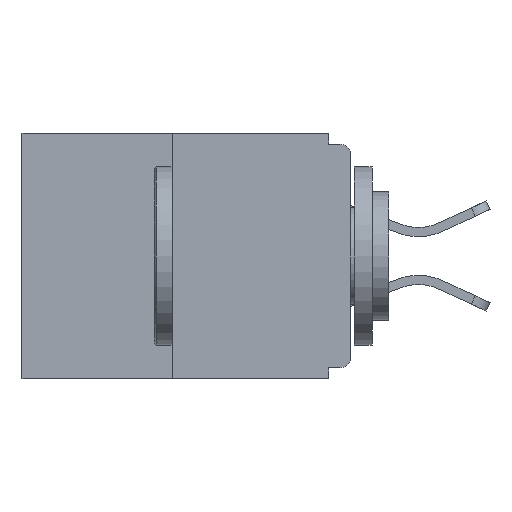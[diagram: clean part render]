
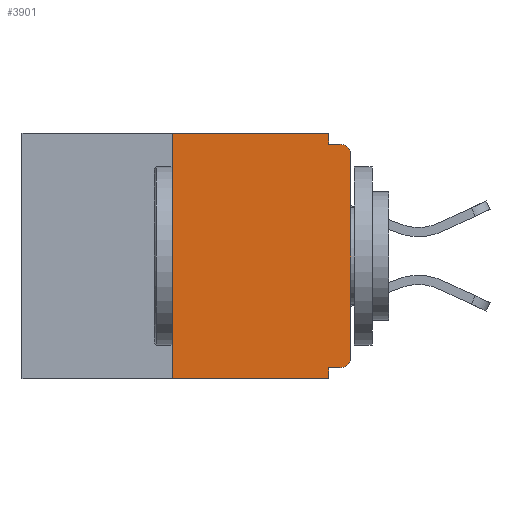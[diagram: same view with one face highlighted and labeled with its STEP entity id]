
A CAD part, left-side view. The second image highlights one B-rep face of the part: STEP entity #3901.
In plain terms, the highlighted planar face has unit normal (-1, 0, 0).
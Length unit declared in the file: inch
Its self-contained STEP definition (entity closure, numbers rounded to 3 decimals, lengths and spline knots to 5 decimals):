
#215 = DIRECTION ( 'NONE',  ( 0., -1., 0. ) ) ;
#288 = CARTESIAN_POINT ( 'NONE',  ( 0., 0.031, -0.015 ) ) ;
#347 = VERTEX_POINT ( 'NONE', #7683 ) ;
#488 = PLANE ( 'NONE',  #17832 ) ;
#621 = VECTOR ( 'NONE', #18661, 39.37008 ) ;
#937 = LINE ( 'NONE', #16950, #2119 ) ;
#1052 = ORIENTED_EDGE ( 'NONE', *, *, #8323, .F. ) ;
#1649 = LINE ( 'NONE', #17513, #13269 ) ;
#1800 = CARTESIAN_POINT ( 'NONE',  ( 0., 0.031, -0.343 ) ) ;
#1850 = EDGE_CURVE ( 'NONE', #15304, #13727, #937, .T. ) ;
#2070 = VERTEX_POINT ( 'NONE', #21611 ) ;
#2119 = VECTOR ( 'NONE', #9263, 39.37008 ) ;
#2448 = DIRECTION ( 'NONE',  ( 1., 0., 0. ) ) ;
#2502 = CARTESIAN_POINT ( 'NONE',  ( 0., 0.015, -0.015 ) ) ;
#2726 = EDGE_CURVE ( 'NONE', #21311, #14760, #7161, .T. ) ;
#2738 = LINE ( 'NONE', #19949, #6299 ) ;
#2855 = ORIENTED_EDGE ( 'NONE', *, *, #10093, .T. ) ;
#3097 = VERTEX_POINT ( 'NONE', #24376 ) ;
#3279 = ORIENTED_EDGE ( 'NONE', *, *, #2726, .T. ) ;
#3549 = EDGE_CURVE ( 'NONE', #15304, #2070, #3857, .T. ) ;
#3606 = ORIENTED_EDGE ( 'NONE', *, *, #1850, .F. ) ;
#3617 = AXIS2_PLACEMENT_3D ( 'NONE', #18743, #9201, #5450 ) ;
#3857 = CIRCLE ( 'NONE', #3617, 0.015 ) ;
#3901 = ADVANCED_FACE ( 'NONE', ( #10687 ), #488, .F. ) ;
#4363 = DIRECTION ( 'NONE',  ( 0., 0., -1. ) ) ;
#4829 = CARTESIAN_POINT ( 'NONE',  ( 0., 0.015, -0.328 ) ) ;
#5216 = AXIS2_PLACEMENT_3D ( 'NONE', #8580, #23591, #8421 ) ;
#5450 = DIRECTION ( 'NONE',  ( 0., 0., -1. ) ) ;
#6033 = ORIENTED_EDGE ( 'NONE', *, *, #14156, .F. ) ;
#6299 = VECTOR ( 'NONE', #20030, 39.37008 ) ;
#6860 = EDGE_CURVE ( 'NONE', #11789, #13066, #14443, .T. ) ;
#7161 = LINE ( 'NONE', #14992, #621 ) ;
#7683 = CARTESIAN_POINT ( 'NONE',  ( 0., 0., -0.03 ) ) ;
#8233 = CARTESIAN_POINT ( 'NONE',  ( 0., 0.031, -0.328 ) ) ;
#8323 = EDGE_CURVE ( 'NONE', #13727, #14760, #18165, .T. ) ;
#8421 = DIRECTION ( 'NONE',  ( 0., 0., -1. ) ) ;
#8580 = CARTESIAN_POINT ( 'NONE',  ( 0., 0.015, -0.03 ) ) ;
#9201 = DIRECTION ( 'NONE',  ( -1., 0., 0. ) ) ;
#9244 = EDGE_CURVE ( 'NONE', #21311, #3097, #2738, .T. ) ;
#9263 = DIRECTION ( 'NONE',  ( 0., 1., 0. ) ) ;
#9691 = CARTESIAN_POINT ( 'NONE',  ( 0., 0., -0.015 ) ) ;
#10093 = EDGE_CURVE ( 'NONE', #2070, #347, #20330, .T. ) ;
#10687 = FACE_OUTER_BOUND ( 'NONE', #21407, .T. ) ;
#10701 = CARTESIAN_POINT ( 'NONE',  ( 0., 0., 0. ) ) ;
#10852 = DIRECTION ( 'NONE',  ( 0., 0., -1. ) ) ;
#11024 = LINE ( 'NONE', #21834, #21178 ) ;
#11789 = VERTEX_POINT ( 'NONE', #288 ) ;
#12007 = VECTOR ( 'NONE', #14549, 39.37008 ) ;
#13066 = VERTEX_POINT ( 'NONE', #2502 ) ;
#13108 = VECTOR ( 'NONE', #10852, 39.37008 ) ;
#13269 = VECTOR ( 'NONE', #13682, 39.37008 ) ;
#13682 = DIRECTION ( 'NONE',  ( 0., -1., 0. ) ) ;
#13727 = VERTEX_POINT ( 'NONE', #8233 ) ;
#14156 = EDGE_CURVE ( 'NONE', #3097, #19572, #1649, .T. ) ;
#14443 = LINE ( 'NONE', #9691, #22787 ) ;
#14452 = ORIENTED_EDGE ( 'NONE', *, *, #20777, .F. ) ;
#14549 = DIRECTION ( 'NONE',  ( 0., 0., 1. ) ) ;
#14760 = VERTEX_POINT ( 'NONE', #1800 ) ;
#14992 = CARTESIAN_POINT ( 'NONE',  ( 0., 0.46, -0.343 ) ) ;
#15304 = VERTEX_POINT ( 'NONE', #4829 ) ;
#15578 = CARTESIAN_POINT ( 'NONE',  ( 0., 0.25, -0.343 ) ) ;
#16950 = CARTESIAN_POINT ( 'NONE',  ( 0., 0., -0.328 ) ) ;
#17513 = CARTESIAN_POINT ( 'NONE',  ( 0., 0.46, 0. ) ) ;
#17552 = CARTESIAN_POINT ( 'NONE',  ( 0., 0.46, 0. ) ) ;
#17832 = AXIS2_PLACEMENT_3D ( 'NONE', #17552, #2448, #4363 ) ;
#17978 = EDGE_CURVE ( 'NONE', #347, #13066, #21890, .T. ) ;
#18165 = LINE ( 'NONE', #22167, #13108 ) ;
#18661 = DIRECTION ( 'NONE',  ( 0., -1., 0. ) ) ;
#18743 = CARTESIAN_POINT ( 'NONE',  ( 0., 0.015, -0.313 ) ) ;
#19572 = VERTEX_POINT ( 'NONE', #20201 ) ;
#19949 = CARTESIAN_POINT ( 'NONE',  ( 0., 0.25, 0. ) ) ;
#20030 = DIRECTION ( 'NONE',  ( 0., 0., 1. ) ) ;
#20201 = CARTESIAN_POINT ( 'NONE',  ( 0., 0.031, 0. ) ) ;
#20330 = LINE ( 'NONE', #10701, #12007 ) ;
#20777 = EDGE_CURVE ( 'NONE', #19572, #11789, #11024, .T. ) ;
#20860 = ORIENTED_EDGE ( 'NONE', *, *, #9244, .F. ) ;
#20880 = ORIENTED_EDGE ( 'NONE', *, *, #17978, .T. ) ;
#21178 = VECTOR ( 'NONE', #23478, 39.37008 ) ;
#21311 = VERTEX_POINT ( 'NONE', #15578 ) ;
#21407 = EDGE_LOOP ( 'NONE', ( #6033, #20860, #3279, #1052, #3606, #21420, #2855, #20880, #23552, #14452 ) ) ;
#21420 = ORIENTED_EDGE ( 'NONE', *, *, #3549, .T. ) ;
#21611 = CARTESIAN_POINT ( 'NONE',  ( 0., 0., -0.313 ) ) ;
#21834 = CARTESIAN_POINT ( 'NONE',  ( 0., 0.031, 0. ) ) ;
#21890 = CIRCLE ( 'NONE', #5216, 0.015 ) ;
#22167 = CARTESIAN_POINT ( 'NONE',  ( 0., 0.031, -0.343 ) ) ;
#22787 = VECTOR ( 'NONE', #215, 39.37008 ) ;
#23478 = DIRECTION ( 'NONE',  ( 0., 0., -1. ) ) ;
#23552 = ORIENTED_EDGE ( 'NONE', *, *, #6860, .F. ) ;
#23591 = DIRECTION ( 'NONE',  ( -1., 0., 0. ) ) ;
#24376 = CARTESIAN_POINT ( 'NONE',  ( 0., 0.25, 0. ) ) ;
